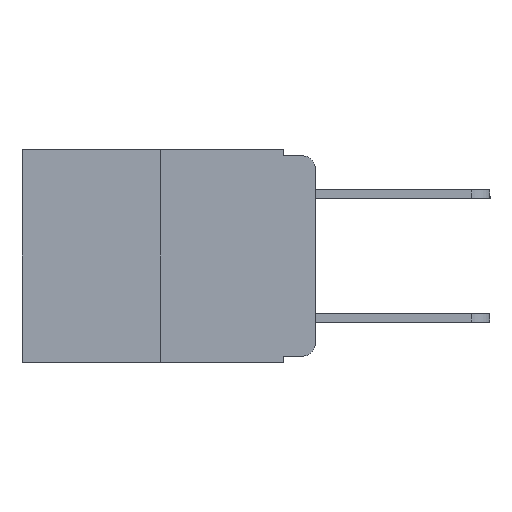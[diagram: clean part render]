
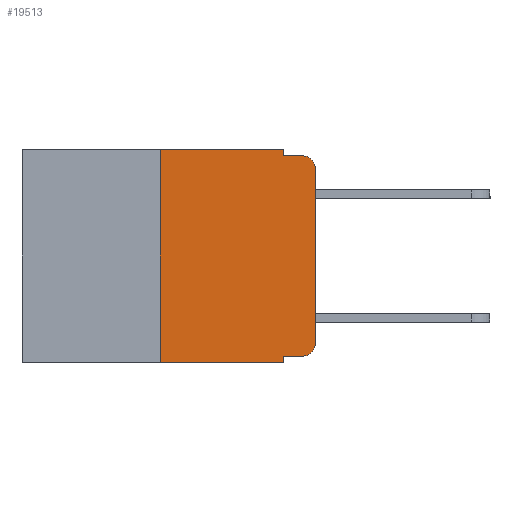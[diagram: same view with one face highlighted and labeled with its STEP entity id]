
A CAD part, left-side view. The second image highlights one B-rep face of the part: STEP entity #19513.
In plain terms, the highlighted planar face has unit normal (-1, 0, 0).
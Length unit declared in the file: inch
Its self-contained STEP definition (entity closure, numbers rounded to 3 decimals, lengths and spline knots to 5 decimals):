
#49 = ORIENTED_EDGE ( 'NONE', *, *, #1640, .T. ) ;
#51 = LINE ( 'NONE', #22457, #694 ) ;
#102 = CARTESIAN_POINT ( 'NONE',  ( 0., 0.02, -0.03 ) ) ;
#128 = VECTOR ( 'NONE', #13839, 39.37008 ) ;
#132 = CARTESIAN_POINT ( 'NONE',  ( 0., 0.25, -0.343 ) ) ;
#694 = VECTOR ( 'NONE', #22535, 39.37008 ) ;
#756 = EDGE_CURVE ( 'NONE', #14215, #24065, #17443, .T. ) ;
#1522 = VECTOR ( 'NONE', #2560, 39.37008 ) ;
#1640 = EDGE_CURVE ( 'NONE', #24065, #2773, #20398, .T. ) ;
#1898 = VERTEX_POINT ( 'NONE', #14125 ) ;
#2192 = DIRECTION ( 'NONE',  ( 0., 0., -1. ) ) ;
#2261 = LINE ( 'NONE', #4244, #21960 ) ;
#2560 = DIRECTION ( 'NONE',  ( 0., 0., -1. ) ) ;
#2773 = VERTEX_POINT ( 'NONE', #19015 ) ;
#2849 = DIRECTION ( 'NONE',  ( 0., 0., 1. ) ) ;
#3674 = ORIENTED_EDGE ( 'NONE', *, *, #10338, .F. ) ;
#4029 = CARTESIAN_POINT ( 'NONE',  ( 0., 0.25, 0. ) ) ;
#4220 = DIRECTION ( 'NONE',  ( 0., 0., -1. ) ) ;
#4244 = CARTESIAN_POINT ( 'NONE',  ( 0., 0.051, -0.333 ) ) ;
#4468 = DIRECTION ( 'NONE',  ( 1., 0., 0. ) ) ;
#4925 = EDGE_CURVE ( 'NONE', #1898, #14215, #2261, .T. ) ;
#5020 = AXIS2_PLACEMENT_3D ( 'NONE', #102, #14171, #2192 ) ;
#5462 = DIRECTION ( 'NONE',  ( 0., -1., 0. ) ) ;
#5568 = CARTESIAN_POINT ( 'NONE',  ( 0., 0.02, -0.313 ) ) ;
#5795 = LINE ( 'NONE', #17276, #16299 ) ;
#6172 = VECTOR ( 'NONE', #25404, 39.37008 ) ;
#6240 = ORIENTED_EDGE ( 'NONE', *, *, #4925, .T. ) ;
#6304 = EDGE_CURVE ( 'NONE', #1898, #7751, #12282, .T. ) ;
#7751 = VERTEX_POINT ( 'NONE', #19685 ) ;
#8905 = CARTESIAN_POINT ( 'NONE',  ( 0., 0.02, -0.333 ) ) ;
#8986 = DIRECTION ( 'NONE',  ( 0., 0., -1. ) ) ;
#9053 = VERTEX_POINT ( 'NONE', #21540 ) ;
#9354 = ORIENTED_EDGE ( 'NONE', *, *, #11652, .F. ) ;
#9377 = ORIENTED_EDGE ( 'NONE', *, *, #6304, .F. ) ;
#9486 = VECTOR ( 'NONE', #2849, 39.37008 ) ;
#9655 = ORIENTED_EDGE ( 'NONE', *, *, #18134, .T. ) ;
#9986 = LINE ( 'NONE', #12077, #6172 ) ;
#9992 = ORIENTED_EDGE ( 'NONE', *, *, #20090, .T. ) ;
#10054 = DIRECTION ( 'NONE',  ( -1., 0., 0. ) ) ;
#10338 = EDGE_CURVE ( 'NONE', #23358, #16258, #51, .T. ) ;
#11652 = EDGE_CURVE ( 'NONE', #21634, #9053, #19973, .T. ) ;
#12077 = CARTESIAN_POINT ( 'NONE',  ( 0., 0.473, -0.343 ) ) ;
#12282 = LINE ( 'NONE', #22633, #1522 ) ;
#13775 = EDGE_CURVE ( 'NONE', #16258, #21634, #5795, .T. ) ;
#13839 = DIRECTION ( 'NONE',  ( 0., -1., 0. ) ) ;
#14023 = CIRCLE ( 'NONE', #5020, 0.02 ) ;
#14125 = CARTESIAN_POINT ( 'NONE',  ( 0., 0.051, -0.333 ) ) ;
#14171 = DIRECTION ( 'NONE',  ( -1., 0., 0. ) ) ;
#14215 = VERTEX_POINT ( 'NONE', #8905 ) ;
#15166 = CARTESIAN_POINT ( 'NONE',  ( 0., 0., -0.313 ) ) ;
#15760 = ORIENTED_EDGE ( 'NONE', *, *, #16843, .F. ) ;
#16130 = LINE ( 'NONE', #25245, #128 ) ;
#16258 = VERTEX_POINT ( 'NONE', #4029 ) ;
#16299 = VECTOR ( 'NONE', #5462, 39.37008 ) ;
#16313 = AXIS2_PLACEMENT_3D ( 'NONE', #23875, #4468, #18264 ) ;
#16843 = EDGE_CURVE ( 'NONE', #9053, #23097, #16130, .T. ) ;
#17276 = CARTESIAN_POINT ( 'NONE',  ( 0., 0.473, 0. ) ) ;
#17372 = CARTESIAN_POINT ( 'NONE',  ( 0., 0.02, -0.01 ) ) ;
#17443 = CIRCLE ( 'NONE', #17872, 0.02 ) ;
#17621 = FACE_OUTER_BOUND ( 'NONE', #23407, .T. ) ;
#17872 = AXIS2_PLACEMENT_3D ( 'NONE', #5568, #10054, #4220 ) ;
#18134 = EDGE_CURVE ( 'NONE', #2773, #23097, #14023, .T. ) ;
#18176 = PLANE ( 'NONE',  #16313 ) ;
#18200 = CARTESIAN_POINT ( 'NONE',  ( 0., 0.051, 0. ) ) ;
#18264 = DIRECTION ( 'NONE',  ( 0., 0., -1. ) ) ;
#18741 = CARTESIAN_POINT ( 'NONE',  ( 0., 0.051, 0. ) ) ;
#19015 = CARTESIAN_POINT ( 'NONE',  ( 0., 0., -0.03 ) ) ;
#19513 = ADVANCED_FACE ( 'NONE', ( #17621 ), #18176, .F. ) ;
#19685 = CARTESIAN_POINT ( 'NONE',  ( 0., 0.051, -0.343 ) ) ;
#19973 = LINE ( 'NONE', #18741, #24358 ) ;
#19982 = ORIENTED_EDGE ( 'NONE', *, *, #13775, .F. ) ;
#20090 = EDGE_CURVE ( 'NONE', #23358, #7751, #9986, .T. ) ;
#20398 = LINE ( 'NONE', #23921, #9486 ) ;
#20405 = DIRECTION ( 'NONE',  ( 0., -1., 0. ) ) ;
#20604 = ORIENTED_EDGE ( 'NONE', *, *, #756, .T. ) ;
#21540 = CARTESIAN_POINT ( 'NONE',  ( 0., 0.051, -0.01 ) ) ;
#21634 = VERTEX_POINT ( 'NONE', #18200 ) ;
#21960 = VECTOR ( 'NONE', #20405, 39.37008 ) ;
#22457 = CARTESIAN_POINT ( 'NONE',  ( 0., 0.25, 0. ) ) ;
#22535 = DIRECTION ( 'NONE',  ( 0., 0., 1. ) ) ;
#22633 = CARTESIAN_POINT ( 'NONE',  ( 0., 0.051, 0. ) ) ;
#23097 = VERTEX_POINT ( 'NONE', #17372 ) ;
#23358 = VERTEX_POINT ( 'NONE', #132 ) ;
#23407 = EDGE_LOOP ( 'NONE', ( #49, #9655, #15760, #9354, #19982, #3674, #9992, #9377, #6240, #20604 ) ) ;
#23875 = CARTESIAN_POINT ( 'NONE',  ( 0., 0.473, 0. ) ) ;
#23921 = CARTESIAN_POINT ( 'NONE',  ( 0., 0., 0. ) ) ;
#24065 = VERTEX_POINT ( 'NONE', #15166 ) ;
#24358 = VECTOR ( 'NONE', #8986, 39.37008 ) ;
#25245 = CARTESIAN_POINT ( 'NONE',  ( 0., 0.051, -0.01 ) ) ;
#25404 = DIRECTION ( 'NONE',  ( 0., -1., 0. ) ) ;
